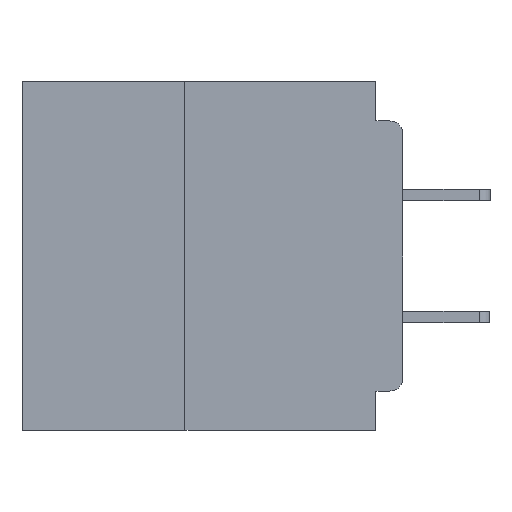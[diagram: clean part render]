
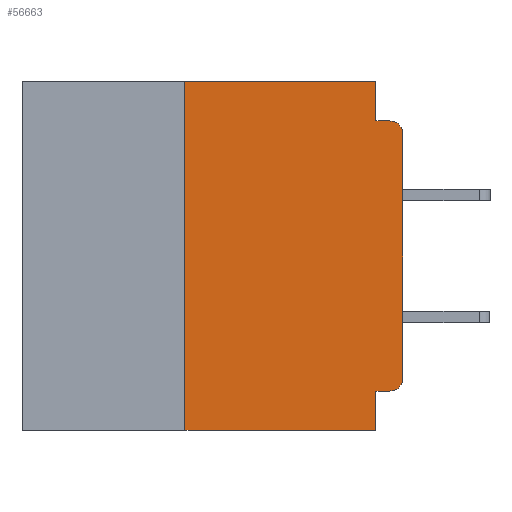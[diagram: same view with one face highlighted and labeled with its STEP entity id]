
A CAD part, left-side view. The second image highlights one B-rep face of the part: STEP entity #56663.
In plain terms, the highlighted planar face has unit normal (-1, 0, 0).
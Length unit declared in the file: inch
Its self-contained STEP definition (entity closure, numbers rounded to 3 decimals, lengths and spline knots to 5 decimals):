
#24 = VECTOR ( 'NONE', #54920, 39.37008 ) ;
#295 = CARTESIAN_POINT ( 'NONE',  ( 0., 0.25, -0.4 ) ) ;
#919 = DIRECTION ( 'NONE',  ( 0., -1., 0. ) ) ;
#2582 = AXIS2_PLACEMENT_3D ( 'NONE', #16790, #21342, #52903 ) ;
#3045 = VECTOR ( 'NONE', #28974, 39.37008 ) ;
#4775 = VECTOR ( 'NONE', #47494, 39.37008 ) ;
#6835 = EDGE_CURVE ( 'NONE', #51315, #18909, #37713, .T. ) ;
#7092 = VERTEX_POINT ( 'NONE', #15986 ) ;
#7212 = CARTESIAN_POINT ( 'NONE',  ( 0., 0., -0.355 ) ) ;
#7300 = ORIENTED_EDGE ( 'NONE', *, *, #22528, .F. ) ;
#8080 = LINE ( 'NONE', #55789, #18769 ) ;
#8297 = DIRECTION ( 'NONE',  ( -1., 0., 0. ) ) ;
#10360 = ORIENTED_EDGE ( 'NONE', *, *, #52709, .T. ) ;
#10555 = DIRECTION ( 'NONE',  ( 0., 0., -1. ) ) ;
#10957 = AXIS2_PLACEMENT_3D ( 'NONE', #15798, #47409, #20371 ) ;
#11705 = CARTESIAN_POINT ( 'NONE',  ( 0., 0.015, -0.045 ) ) ;
#11751 = LINE ( 'NONE', #28246, #22406 ) ;
#12210 = VECTOR ( 'NONE', #44752, 39.37008 ) ;
#12896 = DIRECTION ( 'NONE',  ( 0., -1., 0. ) ) ;
#14203 = FACE_OUTER_BOUND ( 'NONE', #51695, .T. ) ;
#14509 = ORIENTED_EDGE ( 'NONE', *, *, #36890, .T. ) ;
#15518 = CIRCLE ( 'NONE', #35922, 0.015 ) ;
#15798 = CARTESIAN_POINT ( 'NONE',  ( 0., 0.015, -0.34 ) ) ;
#15986 = CARTESIAN_POINT ( 'NONE',  ( 0., 0.015, -0.355 ) ) ;
#16347 = CARTESIAN_POINT ( 'NONE',  ( 0., 0., -0.06 ) ) ;
#16790 = CARTESIAN_POINT ( 'NONE',  ( 0., 0.437, 0. ) ) ;
#18108 = LINE ( 'NONE', #7212, #28692 ) ;
#18370 = LINE ( 'NONE', #29538, #4775 ) ;
#18443 = ORIENTED_EDGE ( 'NONE', *, *, #40260, .F. ) ;
#18769 = VECTOR ( 'NONE', #10555, 39.37008 ) ;
#18909 = VERTEX_POINT ( 'NONE', #47936 ) ;
#20371 = DIRECTION ( 'NONE',  ( 0., 0., -1. ) ) ;
#21342 = DIRECTION ( 'NONE',  ( 1., 0., 0. ) ) ;
#21978 = EDGE_CURVE ( 'NONE', #49987, #28605, #11751, .T. ) ;
#22121 = CARTESIAN_POINT ( 'NONE',  ( 0., 0.25, 0. ) ) ;
#22406 = VECTOR ( 'NONE', #919, 39.37008 ) ;
#22528 = EDGE_CURVE ( 'NONE', #7092, #36073, #18108, .T. ) ;
#25431 = EDGE_CURVE ( 'NONE', #28605, #48558, #18370, .T. ) ;
#28246 = CARTESIAN_POINT ( 'NONE',  ( 0., 0.437, 0. ) ) ;
#28513 = EDGE_CURVE ( 'NONE', #36073, #18909, #8080, .T. ) ;
#28605 = VERTEX_POINT ( 'NONE', #38425 ) ;
#28692 = VECTOR ( 'NONE', #56830, 39.37008 ) ;
#28974 = DIRECTION ( 'NONE',  ( 0., 0., 1. ) ) ;
#29465 = ORIENTED_EDGE ( 'NONE', *, *, #51074, .T. ) ;
#29538 = CARTESIAN_POINT ( 'NONE',  ( 0., 0.031, 0. ) ) ;
#30620 = EDGE_CURVE ( 'NONE', #48558, #39216, #45323, .T. ) ;
#32212 = CARTESIAN_POINT ( 'NONE',  ( 0., 0.437, -0.4 ) ) ;
#33293 = VECTOR ( 'NONE', #12896, 39.37008 ) ;
#35396 = CARTESIAN_POINT ( 'NONE',  ( 0., 0.015, -0.06 ) ) ;
#35922 = AXIS2_PLACEMENT_3D ( 'NONE', #35396, #8297, #39930 ) ;
#36073 = VERTEX_POINT ( 'NONE', #45638 ) ;
#36117 = ORIENTED_EDGE ( 'NONE', *, *, #30620, .F. ) ;
#36890 = EDGE_CURVE ( 'NONE', #58145, #38600, #48300, .T. ) ;
#37713 = LINE ( 'NONE', #32212, #24 ) ;
#38425 = CARTESIAN_POINT ( 'NONE',  ( 0., 0.031, 0. ) ) ;
#38600 = VERTEX_POINT ( 'NONE', #16347 ) ;
#38605 = ORIENTED_EDGE ( 'NONE', *, *, #25431, .F. ) ;
#38800 = CARTESIAN_POINT ( 'NONE',  ( 0., 0., -0.34 ) ) ;
#39216 = VERTEX_POINT ( 'NONE', #11705 ) ;
#39930 = DIRECTION ( 'NONE',  ( 0., 0., -1. ) ) ;
#40206 = CARTESIAN_POINT ( 'NONE',  ( 0., 0., 0. ) ) ;
#40260 = EDGE_CURVE ( 'NONE', #51315, #49987, #51251, .T. ) ;
#40383 = ORIENTED_EDGE ( 'NONE', *, *, #21978, .F. ) ;
#42366 = CARTESIAN_POINT ( 'NONE',  ( 0., 0.25, -0.4 ) ) ;
#43562 = CARTESIAN_POINT ( 'NONE',  ( 0., 0.031, -0.045 ) ) ;
#44752 = DIRECTION ( 'NONE',  ( 0., 0., 1. ) ) ;
#45323 = LINE ( 'NONE', #57952, #33293 ) ;
#45638 = CARTESIAN_POINT ( 'NONE',  ( 0., 0.031, -0.355 ) ) ;
#45814 = ORIENTED_EDGE ( 'NONE', *, *, #6835, .T. ) ;
#47409 = DIRECTION ( 'NONE',  ( -1., 0., 0. ) ) ;
#47494 = DIRECTION ( 'NONE',  ( 0., 0., -1. ) ) ;
#47936 = CARTESIAN_POINT ( 'NONE',  ( 0., 0.031, -0.4 ) ) ;
#48300 = LINE ( 'NONE', #40206, #12210 ) ;
#48558 = VERTEX_POINT ( 'NONE', #43562 ) ;
#49987 = VERTEX_POINT ( 'NONE', #22121 ) ;
#51074 = EDGE_CURVE ( 'NONE', #38600, #39216, #15518, .T. ) ;
#51251 = LINE ( 'NONE', #42366, #3045 ) ;
#51315 = VERTEX_POINT ( 'NONE', #295 ) ;
#51695 = EDGE_LOOP ( 'NONE', ( #14509, #29465, #36117, #38605, #40383, #18443, #45814, #53627, #7300, #10360 ) ) ;
#52709 = EDGE_CURVE ( 'NONE', #7092, #58145, #57014, .T. ) ;
#52903 = DIRECTION ( 'NONE',  ( 0., 0., -1. ) ) ;
#53627 = ORIENTED_EDGE ( 'NONE', *, *, #28513, .F. ) ;
#54920 = DIRECTION ( 'NONE',  ( 0., -1., 0. ) ) ;
#55789 = CARTESIAN_POINT ( 'NONE',  ( 0., 0.031, -0.4 ) ) ;
#56663 = ADVANCED_FACE ( 'NONE', ( #14203 ), #57253, .F. ) ;
#56830 = DIRECTION ( 'NONE',  ( 0., 1., 0. ) ) ;
#57014 = CIRCLE ( 'NONE', #10957, 0.015 ) ;
#57253 = PLANE ( 'NONE',  #2582 ) ;
#57952 = CARTESIAN_POINT ( 'NONE',  ( 0., 0., -0.045 ) ) ;
#58145 = VERTEX_POINT ( 'NONE', #38800 ) ;
